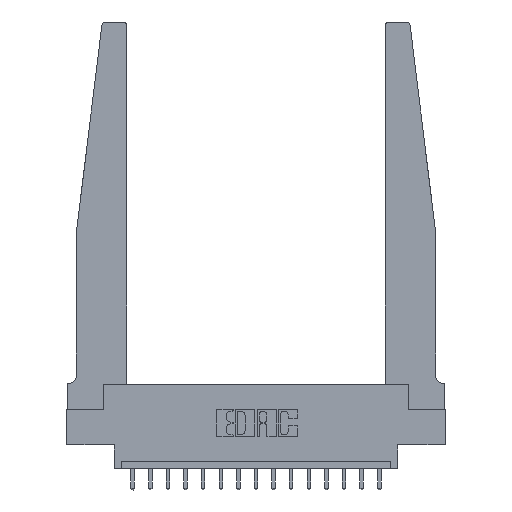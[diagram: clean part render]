
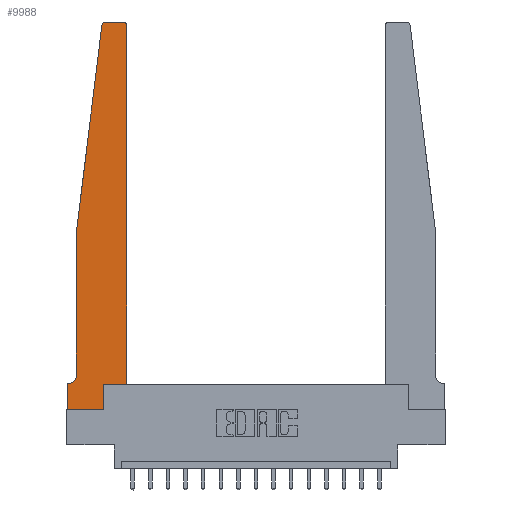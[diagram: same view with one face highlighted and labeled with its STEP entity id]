
A CAD part, top view. The second image highlights one B-rep face of the part: STEP entity #9988.
In plain terms, the highlighted planar face has unit normal (0, 0, 1).
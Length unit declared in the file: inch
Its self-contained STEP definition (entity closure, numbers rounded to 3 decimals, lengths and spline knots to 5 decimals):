
#182 = CARTESIAN_POINT ( 'NONE',  ( 0.065, 1.25, 0.37 ) ) ;
#431 = CARTESIAN_POINT ( 'NONE',  ( 0., 0.1875, 0.37 ) ) ;
#449 = CARTESIAN_POINT ( 'NONE',  ( 0., 0.1875, 0.37 ) ) ;
#496 = AXIS2_PLACEMENT_3D ( 'NONE', #449, #3197, #10055 ) ;
#633 = CARTESIAN_POINT ( 'NONE',  ( 0.27653, 2.75, 0.37 ) ) ;
#666 = VERTEX_POINT ( 'NONE', #8188 ) ;
#788 = CIRCLE ( 'NONE', #16071, 0.05 ) ;
#822 = VERTEX_POINT ( 'NONE', #11588 ) ;
#925 = DIRECTION ( 'NONE',  ( 0., 1., 0. ) ) ;
#963 = ORIENTED_EDGE ( 'NONE', *, *, #6607, .T. ) ;
#1417 = CARTESIAN_POINT ( 'NONE',  ( 0.395, 2.72, 0.37 ) ) ;
#1821 = LINE ( 'NONE', #9062, #2258 ) ;
#1924 = EDGE_CURVE ( 'NONE', #14933, #8049, #15800, .T. ) ;
#2003 = LINE ( 'NONE', #10382, #6111 ) ;
#2125 = VECTOR ( 'NONE', #13609, 39.37008 ) ;
#2199 = DIRECTION ( 'NONE',  ( -1., 0., 0. ) ) ;
#2258 = VECTOR ( 'NONE', #10874, 39.37008 ) ;
#2508 = ORIENTED_EDGE ( 'NONE', *, *, #9272, .T. ) ;
#2609 = CARTESIAN_POINT ( 'NONE',  ( 0.065, 1.25, 0.37 ) ) ;
#2703 = DIRECTION ( 'NONE',  ( 1., 0., 0. ) ) ;
#2767 = DIRECTION ( 'NONE',  ( 0., 0., 1. ) ) ;
#3084 = CARTESIAN_POINT ( 'NONE',  ( 0.2605, 0., 0.37 ) ) ;
#3197 = DIRECTION ( 'NONE',  ( 0., 0., 1. ) ) ;
#3329 = AXIS2_PLACEMENT_3D ( 'NONE', #1417, #2767, #2703 ) ;
#3450 = FACE_OUTER_BOUND ( 'NONE', #8768, .T. ) ;
#3682 = ORIENTED_EDGE ( 'NONE', *, *, #7215, .T. ) ;
#4124 = CARTESIAN_POINT ( 'NONE',  ( 0.24675, 2.72367, 0.37 ) ) ;
#4162 = DIRECTION ( 'NONE',  ( -1., 0., 0. ) ) ;
#4225 = CARTESIAN_POINT ( 'NONE',  ( 0.27653, 2.72, 0.37 ) ) ;
#4259 = EDGE_CURVE ( 'NONE', #10232, #13277, #788, .T. ) ;
#4559 = DIRECTION ( 'NONE',  ( 1., 0., 0. ) ) ;
#4745 = CARTESIAN_POINT ( 'NONE',  ( 0.015, 0.1875, 0.37 ) ) ;
#4784 = VERTEX_POINT ( 'NONE', #4996 ) ;
#4996 = CARTESIAN_POINT ( 'NONE',  ( 0.425, 2.72, 0.37 ) ) ;
#5141 = VERTEX_POINT ( 'NONE', #3084 ) ;
#5493 = DIRECTION ( 'NONE',  ( 0., 0., 1. ) ) ;
#5578 = VECTOR ( 'NONE', #4559, 39.37008 ) ;
#5627 = DIRECTION ( 'NONE',  ( -0.122, -0.992, 0. ) ) ;
#5830 = ORIENTED_EDGE ( 'NONE', *, *, #12389, .T. ) ;
#6099 = EDGE_CURVE ( 'NONE', #16516, #10232, #8422, .T. ) ;
#6111 = VECTOR ( 'NONE', #2199, 39.37008 ) ;
#6607 = EDGE_CURVE ( 'NONE', #666, #17330, #2003, .T. ) ;
#6907 = DIRECTION ( 'NONE',  ( 0., 0., -1. ) ) ;
#7215 = EDGE_CURVE ( 'NONE', #17330, #14558, #13211, .T. ) ;
#7503 = LINE ( 'NONE', #8007, #2125 ) ;
#7821 = VECTOR ( 'NONE', #14308, 39.37008 ) ;
#8007 = CARTESIAN_POINT ( 'NONE',  ( 0.2605, 0.18, 0.37 ) ) ;
#8049 = VERTEX_POINT ( 'NONE', #14984 ) ;
#8074 = VECTOR ( 'NONE', #5627, 39.37008 ) ;
#8188 = CARTESIAN_POINT ( 'NONE',  ( 0.395, 2.75, 0.37 ) ) ;
#8300 = CARTESIAN_POINT ( 'NONE',  ( 0., 0., 0.37 ) ) ;
#8422 = LINE ( 'NONE', #182, #10775 ) ;
#8452 = DIRECTION ( 'NONE',  ( 0., -1., 0. ) ) ;
#8768 = EDGE_LOOP ( 'NONE', ( #963, #3682, #11771, #12579, #17298, #5830, #9778, #13613, #10802, #10929, #2508, #8802 ) ) ;
#8802 = ORIENTED_EDGE ( 'NONE', *, *, #14552, .T. ) ;
#8804 = LINE ( 'NONE', #8300, #13356 ) ;
#9062 = CARTESIAN_POINT ( 'NONE',  ( 0.065, 0.1875, 0.37 ) ) ;
#9272 = EDGE_CURVE ( 'NONE', #10381, #4784, #11425, .T. ) ;
#9502 = EDGE_CURVE ( 'NONE', #8049, #5141, #8804, .T. ) ;
#9507 = DIRECTION ( 'NONE',  ( 1., 0., 0. ) ) ;
#9778 = ORIENTED_EDGE ( 'NONE', *, *, #1924, .T. ) ;
#9818 = AXIS2_PLACEMENT_3D ( 'NONE', #4225, #5493, #9507 ) ;
#9840 = CIRCLE ( 'NONE', #3329, 0.03 ) ;
#9924 = VECTOR ( 'NONE', #925, 39.37008 ) ;
#9988 = ADVANCED_FACE ( 'NONE', ( #3450 ), #9997, .T. ) ;
#9997 = PLANE ( 'NONE',  #496 ) ;
#10055 = DIRECTION ( 'NONE',  ( 1., 0., 0. ) ) ;
#10232 = VERTEX_POINT ( 'NONE', #10659 ) ;
#10381 = VERTEX_POINT ( 'NONE', #14945 ) ;
#10382 = CARTESIAN_POINT ( 'NONE',  ( 0.25, 2.75, 0.37 ) ) ;
#10390 = EDGE_CURVE ( 'NONE', #5141, #822, #7503, .T. ) ;
#10659 = CARTESIAN_POINT ( 'NONE',  ( 0.065, 0.2375, 0.37 ) ) ;
#10775 = VECTOR ( 'NONE', #8452, 39.37008 ) ;
#10802 = ORIENTED_EDGE ( 'NONE', *, *, #10390, .T. ) ;
#10874 = DIRECTION ( 'NONE',  ( -1., 0., 0. ) ) ;
#10929 = ORIENTED_EDGE ( 'NONE', *, *, #11051, .T. ) ;
#11051 = EDGE_CURVE ( 'NONE', #822, #10381, #12679, .T. ) ;
#11425 = LINE ( 'NONE', #11940, #9924 ) ;
#11588 = CARTESIAN_POINT ( 'NONE',  ( 0.2605, 0.18, 0.37 ) ) ;
#11771 = ORIENTED_EDGE ( 'NONE', *, *, #14568, .T. ) ;
#11940 = CARTESIAN_POINT ( 'NONE',  ( 0.425, 0.18, 0.37 ) ) ;
#12373 = CARTESIAN_POINT ( 'NONE',  ( 0.015, 0.2375, 0.37 ) ) ;
#12389 = EDGE_CURVE ( 'NONE', #13277, #14933, #1821, .T. ) ;
#12458 = CARTESIAN_POINT ( 'NONE',  ( 0.065, 1.25, 0.37 ) ) ;
#12579 = ORIENTED_EDGE ( 'NONE', *, *, #6099, .T. ) ;
#12679 = LINE ( 'NONE', #16807, #5578 ) ;
#13211 = CIRCLE ( 'NONE', #9818, 0.03 ) ;
#13277 = VERTEX_POINT ( 'NONE', #4745 ) ;
#13356 = VECTOR ( 'NONE', #15334, 39.37008 ) ;
#13609 = DIRECTION ( 'NONE',  ( 0., 1., 0. ) ) ;
#13613 = ORIENTED_EDGE ( 'NONE', *, *, #9502, .T. ) ;
#14308 = DIRECTION ( 'NONE',  ( 0., -1., 0. ) ) ;
#14552 = EDGE_CURVE ( 'NONE', #4784, #666, #9840, .T. ) ;
#14558 = VERTEX_POINT ( 'NONE', #4124 ) ;
#14568 = EDGE_CURVE ( 'NONE', #14558, #16516, #16481, .T. ) ;
#14933 = VERTEX_POINT ( 'NONE', #431 ) ;
#14945 = CARTESIAN_POINT ( 'NONE',  ( 0.425, 0.18, 0.37 ) ) ;
#14984 = CARTESIAN_POINT ( 'NONE',  ( 0., 0., 0.37 ) ) ;
#15334 = DIRECTION ( 'NONE',  ( 1., 0., 0. ) ) ;
#15589 = CARTESIAN_POINT ( 'NONE',  ( 0., 0., 0.37 ) ) ;
#15800 = LINE ( 'NONE', #15589, #7821 ) ;
#16071 = AXIS2_PLACEMENT_3D ( 'NONE', #12373, #6907, #4162 ) ;
#16481 = LINE ( 'NONE', #12458, #8074 ) ;
#16516 = VERTEX_POINT ( 'NONE', #2609 ) ;
#16807 = CARTESIAN_POINT ( 'NONE',  ( 0.425, 0.18, 0.37 ) ) ;
#17298 = ORIENTED_EDGE ( 'NONE', *, *, #4259, .T. ) ;
#17330 = VERTEX_POINT ( 'NONE', #633 ) ;
